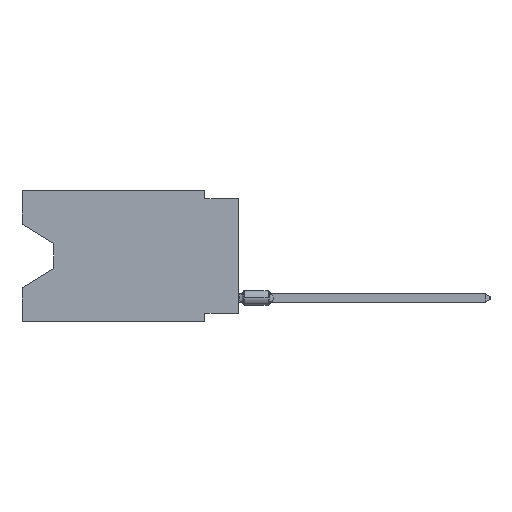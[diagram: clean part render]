
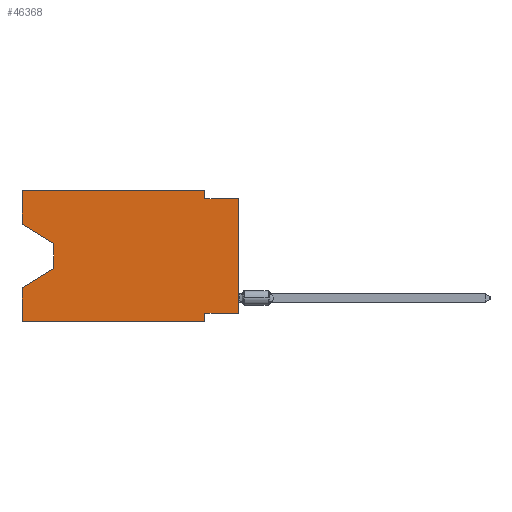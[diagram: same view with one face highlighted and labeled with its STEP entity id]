
A CAD part, left-side view. The second image highlights one B-rep face of the part: STEP entity #46368.
In plain terms, the highlighted planar face has unit normal (-1, 0, 0).
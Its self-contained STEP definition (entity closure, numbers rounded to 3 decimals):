
#118 = VECTOR ( 'NONE', #47435, 1000. ) ;
#600 = CARTESIAN_POINT ( 'NONE',  ( 0., 16.383, -2.546 ) ) ;
#851 = VERTEX_POINT ( 'NONE', #13237 ) ;
#1512 = DIRECTION ( 'NONE',  ( 0., 0., -1. ) ) ;
#2515 = VERTEX_POINT ( 'NONE', #32819 ) ;
#2706 = VERTEX_POINT ( 'NONE', #29990 ) ;
#3887 = DIRECTION ( 'NONE',  ( 0., -1., 0. ) ) ;
#4731 = EDGE_CURVE ( 'NONE', #17610, #40270, #15452, .T. ) ;
#6061 = CARTESIAN_POINT ( 'NONE',  ( 0., 0., -0.635 ) ) ;
#7703 = LINE ( 'NONE', #35874, #47405 ) ;
#8153 = VECTOR ( 'NONE', #8893, 1000. ) ;
#8324 = EDGE_LOOP ( 'NONE', ( #46491, #43750, #25121, #21139, #14473, #44767, #21164, #29481, #43933, #11179, #25575, #45275 ) ) ;
#8325 = DIRECTION ( 'NONE',  ( 0., 0., -1. ) ) ;
#8573 = DIRECTION ( 'NONE',  ( 1., 0., 0. ) ) ;
#8893 = DIRECTION ( 'NONE',  ( 0., 0.855, -0.519 ) ) ;
#10673 = DIRECTION ( 'NONE',  ( 0., 0., 1. ) ) ;
#10819 = CARTESIAN_POINT ( 'NONE',  ( 0., 2.54, -0.635 ) ) ;
#11179 = ORIENTED_EDGE ( 'NONE', *, *, #39301, .F. ) ;
#11972 = LINE ( 'NONE', #39412, #18040 ) ;
#12187 = FACE_OUTER_BOUND ( 'NONE', #8324, .T. ) ;
#13237 = CARTESIAN_POINT ( 'NONE',  ( 0., 2.54, -9.271 ) ) ;
#14218 = VECTOR ( 'NONE', #1512, 1000. ) ;
#14445 = DIRECTION ( 'NONE',  ( 0., 0., 1. ) ) ;
#14473 = ORIENTED_EDGE ( 'NONE', *, *, #20506, .T. ) ;
#15452 = LINE ( 'NONE', #600, #26937 ) ;
#15701 = DIRECTION ( 'NONE',  ( 0., 0., -1. ) ) ;
#16478 = VERTEX_POINT ( 'NONE', #18628 ) ;
#16681 = CARTESIAN_POINT ( 'NONE',  ( 0., 2.54, -9.906 ) ) ;
#17610 = VERTEX_POINT ( 'NONE', #37768 ) ;
#18040 = VECTOR ( 'NONE', #50550, 1000. ) ;
#18200 = EDGE_CURVE ( 'NONE', #851, #43552, #7703, .T. ) ;
#18216 = LINE ( 'NONE', #6061, #23528 ) ;
#18394 = CARTESIAN_POINT ( 'NONE',  ( 0., 0., -0.635 ) ) ;
#18628 = CARTESIAN_POINT ( 'NONE',  ( 0., 16.383, -7.36 ) ) ;
#18650 = EDGE_CURVE ( 'NONE', #17610, #2515, #41873, .T. ) ;
#18949 = DIRECTION ( 'NONE',  ( 0., 0., 1. ) ) ;
#19478 = CARTESIAN_POINT ( 'NONE',  ( 0., 13.97, -5.893 ) ) ;
#19527 = LINE ( 'NONE', #39179, #118 ) ;
#19850 = VERTEX_POINT ( 'NONE', #10819 ) ;
#20137 = CARTESIAN_POINT ( 'NONE',  ( 0., 16.383, -9.906 ) ) ;
#20506 = EDGE_CURVE ( 'NONE', #35390, #43552, #31810, .T. ) ;
#21139 = ORIENTED_EDGE ( 'NONE', *, *, #28650, .F. ) ;
#21164 = ORIENTED_EDGE ( 'NONE', *, *, #43780, .F. ) ;
#21533 = EDGE_CURVE ( 'NONE', #46153, #16478, #28554, .T. ) ;
#22586 = CARTESIAN_POINT ( 'NONE',  ( 0., 2.54, 0. ) ) ;
#22835 = CARTESIAN_POINT ( 'NONE',  ( 0., 0., 0. ) ) ;
#23492 = VERTEX_POINT ( 'NONE', #18394 ) ;
#23528 = VECTOR ( 'NONE', #49773, 1000. ) ;
#24797 = CARTESIAN_POINT ( 'NONE',  ( 0., 2.54, 0. ) ) ;
#25121 = ORIENTED_EDGE ( 'NONE', *, *, #21533, .T. ) ;
#25210 = VECTOR ( 'NONE', #36804, 1000. ) ;
#25575 = ORIENTED_EDGE ( 'NONE', *, *, #30300, .F. ) ;
#26467 = CARTESIAN_POINT ( 'NONE',  ( 0., 16.383, 0. ) ) ;
#26937 = VECTOR ( 'NONE', #36576, 1000. ) ;
#27332 = VECTOR ( 'NONE', #10673, 1000. ) ;
#27976 = PLANE ( 'NONE',  #40037 ) ;
#28451 = VECTOR ( 'NONE', #14445, 1000. ) ;
#28554 = LINE ( 'NONE', #44356, #8153 ) ;
#28650 = EDGE_CURVE ( 'NONE', #35390, #16478, #38612, .T. ) ;
#29481 = ORIENTED_EDGE ( 'NONE', *, *, #41887, .T. ) ;
#29990 = CARTESIAN_POINT ( 'NONE',  ( 0., 0., -9.271 ) ) ;
#30300 = EDGE_CURVE ( 'NONE', #2515, #43006, #19527, .T. ) ;
#31810 = LINE ( 'NONE', #32305, #36949 ) ;
#32142 = CARTESIAN_POINT ( 'NONE',  ( 0., 13.97, -4.013 ) ) ;
#32278 = EDGE_CURVE ( 'NONE', #19850, #23492, #18216, .T. ) ;
#32305 = CARTESIAN_POINT ( 'NONE',  ( 0., 16.383, -9.906 ) ) ;
#32443 = EDGE_CURVE ( 'NONE', #40270, #46153, #48172, .T. ) ;
#32819 = CARTESIAN_POINT ( 'NONE',  ( 0., 16.383, 0. ) ) ;
#35390 = VERTEX_POINT ( 'NONE', #20137 ) ;
#35874 = CARTESIAN_POINT ( 'NONE',  ( 0., 2.54, -9.906 ) ) ;
#36576 = DIRECTION ( 'NONE',  ( 0., -0.855, -0.519 ) ) ;
#36804 = DIRECTION ( 'NONE',  ( 0., 0., -1. ) ) ;
#36949 = VECTOR ( 'NONE', #3887, 1000. ) ;
#37768 = CARTESIAN_POINT ( 'NONE',  ( 0., 16.383, -2.546 ) ) ;
#38612 = LINE ( 'NONE', #26467, #27332 ) ;
#38755 = CARTESIAN_POINT ( 'NONE',  ( 0., 16.383, 0. ) ) ;
#39179 = CARTESIAN_POINT ( 'NONE',  ( 0., 16.383, 0. ) ) ;
#39301 = EDGE_CURVE ( 'NONE', #43006, #19850, #45241, .T. ) ;
#39412 = CARTESIAN_POINT ( 'NONE',  ( 0., 0., -9.271 ) ) ;
#40037 = AXIS2_PLACEMENT_3D ( 'NONE', #44032, #8573, #8325 ) ;
#40270 = VERTEX_POINT ( 'NONE', #48801 ) ;
#41873 = LINE ( 'NONE', #38755, #28451 ) ;
#41887 = EDGE_CURVE ( 'NONE', #2706, #23492, #42497, .T. ) ;
#42497 = LINE ( 'NONE', #22835, #49138 ) ;
#43006 = VERTEX_POINT ( 'NONE', #22586 ) ;
#43552 = VERTEX_POINT ( 'NONE', #16681 ) ;
#43750 = ORIENTED_EDGE ( 'NONE', *, *, #32443, .T. ) ;
#43780 = EDGE_CURVE ( 'NONE', #2706, #851, #11972, .T. ) ;
#43933 = ORIENTED_EDGE ( 'NONE', *, *, #32278, .F. ) ;
#44032 = CARTESIAN_POINT ( 'NONE',  ( 0., 16.383, 0. ) ) ;
#44356 = CARTESIAN_POINT ( 'NONE',  ( 0., 13.97, -5.893 ) ) ;
#44767 = ORIENTED_EDGE ( 'NONE', *, *, #18200, .F. ) ;
#45241 = LINE ( 'NONE', #24797, #14218 ) ;
#45275 = ORIENTED_EDGE ( 'NONE', *, *, #18650, .F. ) ;
#46153 = VERTEX_POINT ( 'NONE', #19478 ) ;
#46368 = ADVANCED_FACE ( 'NONE', ( #12187 ), #27976, .F. ) ;
#46491 = ORIENTED_EDGE ( 'NONE', *, *, #4731, .T. ) ;
#47405 = VECTOR ( 'NONE', #15701, 1000. ) ;
#47435 = DIRECTION ( 'NONE',  ( 0., -1., 0. ) ) ;
#48172 = LINE ( 'NONE', #32142, #25210 ) ;
#48801 = CARTESIAN_POINT ( 'NONE',  ( 0., 13.97, -4.013 ) ) ;
#49138 = VECTOR ( 'NONE', #18949, 1000. ) ;
#49773 = DIRECTION ( 'NONE',  ( 0., -1., 0. ) ) ;
#50550 = DIRECTION ( 'NONE',  ( 0., 1., 0. ) ) ;
